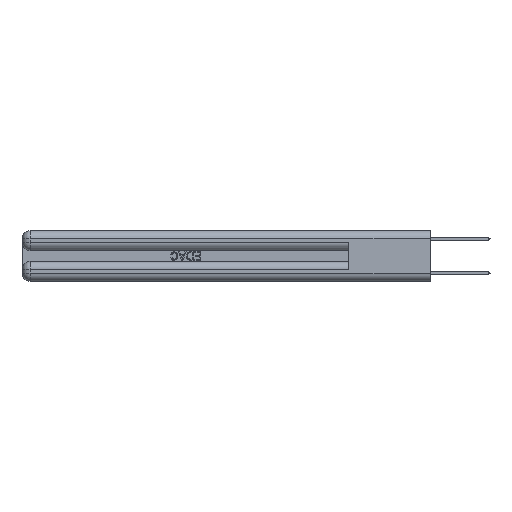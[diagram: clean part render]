
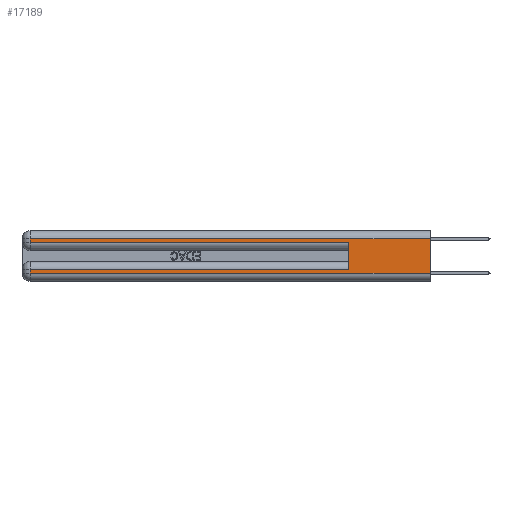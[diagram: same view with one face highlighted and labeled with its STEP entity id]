
A CAD part, left-side view. The second image highlights one B-rep face of the part: STEP entity #17189.
In plain terms, the highlighted planar face has unit normal (-1, 0, 0).
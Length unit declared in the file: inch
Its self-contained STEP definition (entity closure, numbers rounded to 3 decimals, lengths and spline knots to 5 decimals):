
#338 = CARTESIAN_POINT ( 'NONE',  ( 0., 2.94, 0.37 ) ) ;
#637 = LINE ( 'NONE', #3118, #11901 ) ;
#969 = CARTESIAN_POINT ( 'NONE',  ( 0., 2.94, 0.06 ) ) ;
#1643 = VERTEX_POINT ( 'NONE', #28955 ) ;
#1984 = DIRECTION ( 'NONE',  ( 0., -1., 0. ) ) ;
#3058 = DIRECTION ( 'NONE',  ( 0., 0., 1. ) ) ;
#3118 = CARTESIAN_POINT ( 'NONE',  ( 0., 0., 0.31 ) ) ;
#3289 = DIRECTION ( 'NONE',  ( 0., -1., 0. ) ) ;
#3414 = DIRECTION ( 'NONE',  ( 0., 1., 0. ) ) ;
#3609 = ORIENTED_EDGE ( 'NONE', *, *, #8116, .T. ) ;
#3750 = LINE ( 'NONE', #13155, #21110 ) ;
#4074 = LINE ( 'NONE', #22852, #13722 ) ;
#4092 = VERTEX_POINT ( 'NONE', #969 ) ;
#4184 = VECTOR ( 'NONE', #1984, 39.37008 ) ;
#7316 = VECTOR ( 'NONE', #11928, 39.37008 ) ;
#7442 = CARTESIAN_POINT ( 'NONE',  ( 0., 0., 0.06 ) ) ;
#8116 = EDGE_CURVE ( 'NONE', #4092, #21086, #18326, .T. ) ;
#8155 = LINE ( 'NONE', #10168, #26953 ) ;
#8200 = VECTOR ( 'NONE', #12553, 39.37008 ) ;
#8311 = ORIENTED_EDGE ( 'NONE', *, *, #17310, .T. ) ;
#8423 = VERTEX_POINT ( 'NONE', #29974 ) ;
#9246 = VERTEX_POINT ( 'NONE', #12525 ) ;
#9461 = ORIENTED_EDGE ( 'NONE', *, *, #24665, .T. ) ;
#10168 = CARTESIAN_POINT ( 'NONE',  ( 0., 0.6, 0.145 ) ) ;
#10250 = CARTESIAN_POINT ( 'NONE',  ( 0., 0., 0.37 ) ) ;
#10329 = VERTEX_POINT ( 'NONE', #13407 ) ;
#10623 = VERTEX_POINT ( 'NONE', #13072 ) ;
#11157 = ORIENTED_EDGE ( 'NONE', *, *, #17790, .F. ) ;
#11901 = VECTOR ( 'NONE', #3414, 39.37008 ) ;
#11928 = DIRECTION ( 'NONE',  ( 0., 0., -1. ) ) ;
#12333 = CARTESIAN_POINT ( 'NONE',  ( 0., 2.94, 0.37 ) ) ;
#12525 = CARTESIAN_POINT ( 'NONE',  ( 0., 0.6, 0.285 ) ) ;
#12553 = DIRECTION ( 'NONE',  ( 0., 0., -1. ) ) ;
#12603 = EDGE_CURVE ( 'NONE', #10329, #9246, #3750, .T. ) ;
#13072 = CARTESIAN_POINT ( 'NONE',  ( 0., 0.6, 0.085 ) ) ;
#13155 = CARTESIAN_POINT ( 'NONE',  ( 0., 0., 0.285 ) ) ;
#13407 = CARTESIAN_POINT ( 'NONE',  ( 0., 2.94, 0.285 ) ) ;
#13559 = FACE_OUTER_BOUND ( 'NONE', #24637, .T. ) ;
#13562 = AXIS2_PLACEMENT_3D ( 'NONE', #22942, #21091, #20625 ) ;
#13722 = VECTOR ( 'NONE', #30267, 39.37008 ) ;
#16385 = CARTESIAN_POINT ( 'NONE',  ( 0., 2.94, 0.31 ) ) ;
#17189 = ADVANCED_FACE ( 'NONE', ( #13559 ), #18786, .F. ) ;
#17310 = EDGE_CURVE ( 'NONE', #30392, #10329, #26184, .T. ) ;
#17790 = EDGE_CURVE ( 'NONE', #1643, #21086, #29333, .T. ) ;
#18326 = LINE ( 'NONE', #20488, #4184 ) ;
#18786 = PLANE ( 'NONE',  #13562 ) ;
#19287 = ORIENTED_EDGE ( 'NONE', *, *, #12603, .T. ) ;
#19304 = LINE ( 'NONE', #338, #7316 ) ;
#19479 = VECTOR ( 'NONE', #26332, 39.37008 ) ;
#20488 = CARTESIAN_POINT ( 'NONE',  ( 0., 0., 0.06 ) ) ;
#20625 = DIRECTION ( 'NONE',  ( 0., 0., -1. ) ) ;
#21086 = VERTEX_POINT ( 'NONE', #7442 ) ;
#21091 = DIRECTION ( 'NONE',  ( 1., 0., 0. ) ) ;
#21110 = VECTOR ( 'NONE', #3289, 39.37008 ) ;
#21638 = EDGE_CURVE ( 'NONE', #10623, #9246, #8155, .T. ) ;
#21951 = ORIENTED_EDGE ( 'NONE', *, *, #27378, .T. ) ;
#22264 = EDGE_CURVE ( 'NONE', #8423, #4092, #19304, .T. ) ;
#22852 = CARTESIAN_POINT ( 'NONE',  ( 0., 0., 0.085 ) ) ;
#22942 = CARTESIAN_POINT ( 'NONE',  ( 0., 0., 0.37 ) ) ;
#24396 = ORIENTED_EDGE ( 'NONE', *, *, #21638, .F. ) ;
#24637 = EDGE_LOOP ( 'NONE', ( #11157, #21951, #8311, #19287, #24396, #9461, #30406, #3609 ) ) ;
#24665 = EDGE_CURVE ( 'NONE', #10623, #8423, #4074, .T. ) ;
#26184 = LINE ( 'NONE', #12333, #19479 ) ;
#26332 = DIRECTION ( 'NONE',  ( 0., 0., -1. ) ) ;
#26953 = VECTOR ( 'NONE', #3058, 39.37008 ) ;
#27378 = EDGE_CURVE ( 'NONE', #1643, #30392, #637, .T. ) ;
#28955 = CARTESIAN_POINT ( 'NONE',  ( 0., 0., 0.31 ) ) ;
#29333 = LINE ( 'NONE', #10250, #8200 ) ;
#29974 = CARTESIAN_POINT ( 'NONE',  ( 0., 2.94, 0.085 ) ) ;
#30267 = DIRECTION ( 'NONE',  ( 0., 1., 0. ) ) ;
#30392 = VERTEX_POINT ( 'NONE', #16385 ) ;
#30406 = ORIENTED_EDGE ( 'NONE', *, *, #22264, .T. ) ;
